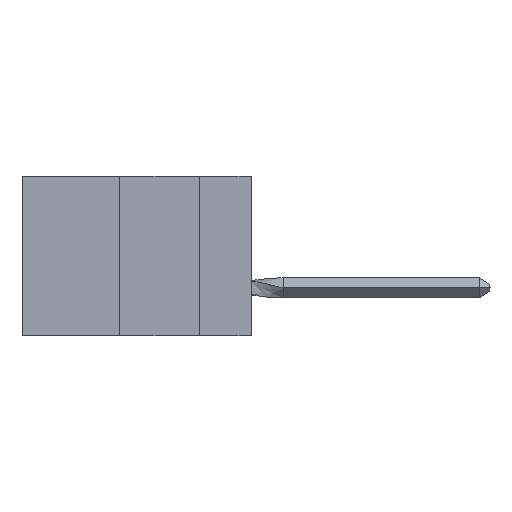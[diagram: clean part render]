
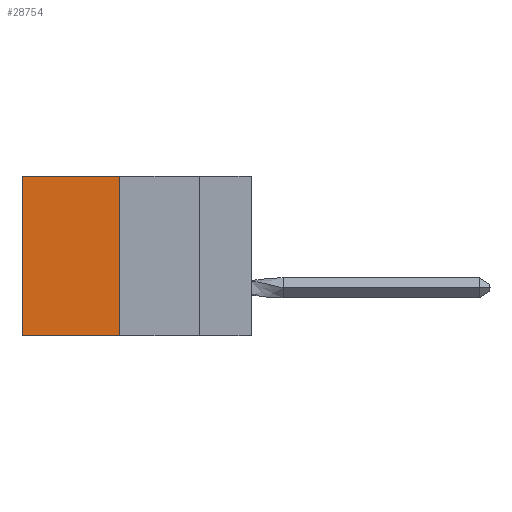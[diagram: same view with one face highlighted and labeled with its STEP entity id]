
A CAD part, left-side view. The second image highlights one B-rep face of the part: STEP entity #28754.
In plain terms, the highlighted planar face has unit normal (-1, 0, 0).
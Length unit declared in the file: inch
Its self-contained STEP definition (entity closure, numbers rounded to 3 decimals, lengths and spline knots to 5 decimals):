
#183 = DIRECTION ( 'NONE',  ( 0., 0., -1. ) ) ;
#1060 = CARTESIAN_POINT ( 'NONE',  ( 0.305, 0.413, -0.5 ) ) ;
#1973 = LINE ( 'NONE', #9350, #24796 ) ;
#2428 = PLANE ( 'NONE',  #4759 ) ;
#2708 = VERTEX_POINT ( 'NONE', #14623 ) ;
#3669 = VERTEX_POINT ( 'NONE', #16687 ) ;
#4759 = AXIS2_PLACEMENT_3D ( 'NONE', #22212, #9685, #183 ) ;
#5423 = EDGE_CURVE ( 'NONE', #11737, #19563, #8242, .T. ) ;
#5506 = CARTESIAN_POINT ( 'NONE',  ( 0.305, 0.72, 0. ) ) ;
#8242 = LINE ( 'NONE', #11889, #12049 ) ;
#9350 = CARTESIAN_POINT ( 'NONE',  ( 0.305, 0.413, 0. ) ) ;
#9356 = FACE_OUTER_BOUND ( 'NONE', #17553, .T. ) ;
#9685 = DIRECTION ( 'NONE',  ( 1., 0., 0. ) ) ;
#9752 = EDGE_CURVE ( 'NONE', #2708, #11737, #1973, .T. ) ;
#9787 = LINE ( 'NONE', #26353, #29137 ) ;
#9882 = ORIENTED_EDGE ( 'NONE', *, *, #24472, .F. ) ;
#11737 = VERTEX_POINT ( 'NONE', #5506 ) ;
#11889 = CARTESIAN_POINT ( 'NONE',  ( 0.305, 0.72, -0.5 ) ) ;
#12049 = VECTOR ( 'NONE', #14030, 39.37008 ) ;
#14030 = DIRECTION ( 'NONE',  ( 0., 0., -1. ) ) ;
#14623 = CARTESIAN_POINT ( 'NONE',  ( 0.305, 0.413, 0. ) ) ;
#16687 = CARTESIAN_POINT ( 'NONE',  ( 0.305, 0.413, -0.5 ) ) ;
#17333 = LINE ( 'NONE', #1060, #26076 ) ;
#17553 = EDGE_LOOP ( 'NONE', ( #24921, #27744, #9882, #23299 ) ) ;
#18085 = DIRECTION ( 'NONE',  ( 0., 0., -1. ) ) ;
#19563 = VERTEX_POINT ( 'NONE', #28207 ) ;
#20120 = EDGE_CURVE ( 'NONE', #3669, #19563, #9787, .T. ) ;
#22212 = CARTESIAN_POINT ( 'NONE',  ( 0.305, 0.413, -0.5 ) ) ;
#23299 = ORIENTED_EDGE ( 'NONE', *, *, #9752, .T. ) ;
#24472 = EDGE_CURVE ( 'NONE', #2708, #3669, #17333, .T. ) ;
#24796 = VECTOR ( 'NONE', #31143, 39.37008 ) ;
#24921 = ORIENTED_EDGE ( 'NONE', *, *, #5423, .T. ) ;
#25934 = DIRECTION ( 'NONE',  ( 0., 1., 0. ) ) ;
#26076 = VECTOR ( 'NONE', #18085, 39.37008 ) ;
#26353 = CARTESIAN_POINT ( 'NONE',  ( 0.305, 0.413, -0.5 ) ) ;
#27744 = ORIENTED_EDGE ( 'NONE', *, *, #20120, .F. ) ;
#28207 = CARTESIAN_POINT ( 'NONE',  ( 0.305, 0.72, -0.5 ) ) ;
#28754 = ADVANCED_FACE ( 'NONE', ( #9356 ), #2428, .F. ) ;
#29137 = VECTOR ( 'NONE', #25934, 39.37008 ) ;
#31143 = DIRECTION ( 'NONE',  ( 0., 1., 0. ) ) ;
